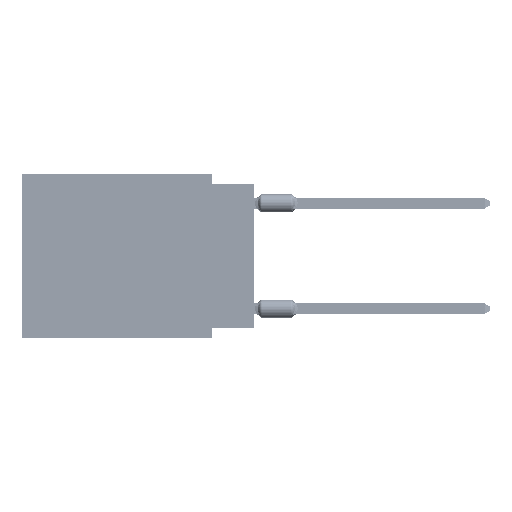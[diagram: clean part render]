
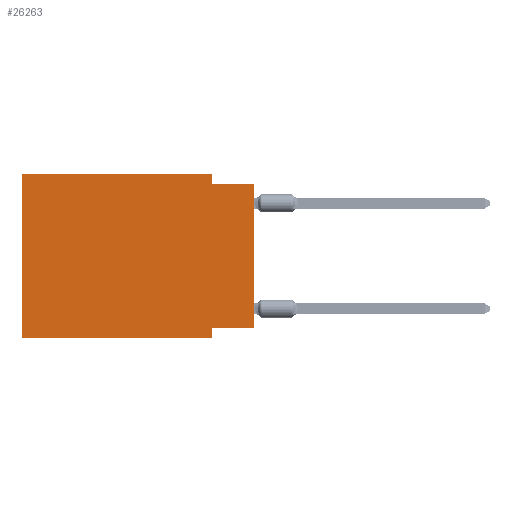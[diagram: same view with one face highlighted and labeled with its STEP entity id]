
A CAD part, left-side view. The second image highlights one B-rep face of the part: STEP entity #26263.
In plain terms, the highlighted planar face has unit normal (-1, 0, 0).
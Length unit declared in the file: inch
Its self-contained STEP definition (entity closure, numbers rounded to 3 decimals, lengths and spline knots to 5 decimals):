
#173 = VECTOR ( 'NONE', #6157, 39.37008 ) ;
#2948 = VECTOR ( 'NONE', #68541, 39.37008 ) ;
#3236 = CARTESIAN_POINT ( 'NONE',  ( 0., 0.1, -0.025 ) ) ;
#4439 = CARTESIAN_POINT ( 'NONE',  ( 0., 0.1, 0. ) ) ;
#4794 = DIRECTION ( 'NONE',  ( 0., 0., -1. ) ) ;
#6099 = CARTESIAN_POINT ( 'NONE',  ( 0., 0.1, -0.39 ) ) ;
#6157 = DIRECTION ( 'NONE',  ( 0., 0., -1. ) ) ;
#6306 = VERTEX_POINT ( 'NONE', #61136 ) ;
#6766 = DIRECTION ( 'NONE',  ( 0., 1., 0. ) ) ;
#6955 = ORIENTED_EDGE ( 'NONE', *, *, #58393, .F. ) ;
#7445 = DIRECTION ( 'NONE',  ( 0., -1., 0. ) ) ;
#7978 = EDGE_CURVE ( 'NONE', #6306, #11005, #34181, .T. ) ;
#9867 = EDGE_LOOP ( 'NONE', ( #35919, #54775, #21187, #40777, #33860, #21230, #6955, #64903 ) ) ;
#10361 = CARTESIAN_POINT ( 'NONE',  ( 0., 0.1, -0.39 ) ) ;
#11005 = VERTEX_POINT ( 'NONE', #42555 ) ;
#13426 = LINE ( 'NONE', #62662, #41597 ) ;
#15803 = CARTESIAN_POINT ( 'NONE',  ( 0., 0.55, -0.39 ) ) ;
#17256 = LINE ( 'NONE', #33321, #49756 ) ;
#18840 = PLANE ( 'NONE',  #37641 ) ;
#19458 = CARTESIAN_POINT ( 'NONE',  ( 0., 0.55, 0. ) ) ;
#21187 = ORIENTED_EDGE ( 'NONE', *, *, #64547, .F. ) ;
#21230 = ORIENTED_EDGE ( 'NONE', *, *, #45893, .T. ) ;
#25602 = CARTESIAN_POINT ( 'NONE',  ( 0., 0.1, 0. ) ) ;
#26263 = ADVANCED_FACE ( 'NONE', ( #66688 ), #18840, .F. ) ;
#28621 = DIRECTION ( 'NONE',  ( 0., 0., 1. ) ) ;
#29848 = DIRECTION ( 'NONE',  ( 0., -1., 0. ) ) ;
#29987 = DIRECTION ( 'NONE',  ( 0., 0., 1. ) ) ;
#30860 = EDGE_CURVE ( 'NONE', #66133, #34839, #49229, .T. ) ;
#33321 = CARTESIAN_POINT ( 'NONE',  ( 0., 0., -0.025 ) ) ;
#33860 = ORIENTED_EDGE ( 'NONE', *, *, #30860, .F. ) ;
#34181 = LINE ( 'NONE', #51285, #42234 ) ;
#34839 = VERTEX_POINT ( 'NONE', #19458 ) ;
#34917 = DIRECTION ( 'NONE',  ( 1., 0., 0. ) ) ;
#35919 = ORIENTED_EDGE ( 'NONE', *, *, #7978, .T. ) ;
#37068 = VECTOR ( 'NONE', #6766, 39.37008 ) ;
#37641 = AXIS2_PLACEMENT_3D ( 'NONE', #40149, #34917, #56207 ) ;
#40149 = CARTESIAN_POINT ( 'NONE',  ( 0., 0.55, 0. ) ) ;
#40777 = ORIENTED_EDGE ( 'NONE', *, *, #66676, .F. ) ;
#41380 = VERTEX_POINT ( 'NONE', #3236 ) ;
#41597 = VECTOR ( 'NONE', #29848, 39.37008 ) ;
#41960 = CARTESIAN_POINT ( 'NONE',  ( 0., 0.55, -0.39 ) ) ;
#42178 = VERTEX_POINT ( 'NONE', #6099 ) ;
#42234 = VECTOR ( 'NONE', #29987, 39.37008 ) ;
#42555 = CARTESIAN_POINT ( 'NONE',  ( 0., 0., -0.025 ) ) ;
#45661 = EDGE_CURVE ( 'NONE', #41380, #11005, #17256, .T. ) ;
#45893 = EDGE_CURVE ( 'NONE', #66133, #42178, #47586, .T. ) ;
#45926 = VERTEX_POINT ( 'NONE', #25602 ) ;
#47586 = LINE ( 'NONE', #15803, #2948 ) ;
#47731 = LINE ( 'NONE', #10361, #173 ) ;
#49229 = LINE ( 'NONE', #49562, #62560 ) ;
#49562 = CARTESIAN_POINT ( 'NONE',  ( 0., 0.55, 0. ) ) ;
#49756 = VECTOR ( 'NONE', #7445, 39.37008 ) ;
#50379 = LINE ( 'NONE', #54587, #37068 ) ;
#50839 = VERTEX_POINT ( 'NONE', #56935 ) ;
#51285 = CARTESIAN_POINT ( 'NONE',  ( 0., 0., 0. ) ) ;
#51930 = LINE ( 'NONE', #4439, #65257 ) ;
#54587 = CARTESIAN_POINT ( 'NONE',  ( 0., 0., -0.365 ) ) ;
#54775 = ORIENTED_EDGE ( 'NONE', *, *, #45661, .F. ) ;
#56207 = DIRECTION ( 'NONE',  ( 0., 0., -1. ) ) ;
#56935 = CARTESIAN_POINT ( 'NONE',  ( 0., 0.1, -0.365 ) ) ;
#58393 = EDGE_CURVE ( 'NONE', #50839, #42178, #47731, .T. ) ;
#59039 = EDGE_CURVE ( 'NONE', #6306, #50839, #50379, .T. ) ;
#61136 = CARTESIAN_POINT ( 'NONE',  ( 0., 0., -0.365 ) ) ;
#62560 = VECTOR ( 'NONE', #28621, 39.37008 ) ;
#62662 = CARTESIAN_POINT ( 'NONE',  ( 0., 0.55, 0. ) ) ;
#64547 = EDGE_CURVE ( 'NONE', #45926, #41380, #51930, .T. ) ;
#64903 = ORIENTED_EDGE ( 'NONE', *, *, #59039, .F. ) ;
#65257 = VECTOR ( 'NONE', #4794, 39.37008 ) ;
#66133 = VERTEX_POINT ( 'NONE', #41960 ) ;
#66676 = EDGE_CURVE ( 'NONE', #34839, #45926, #13426, .T. ) ;
#66688 = FACE_OUTER_BOUND ( 'NONE', #9867, .T. ) ;
#68541 = DIRECTION ( 'NONE',  ( 0., -1., 0. ) ) ;
